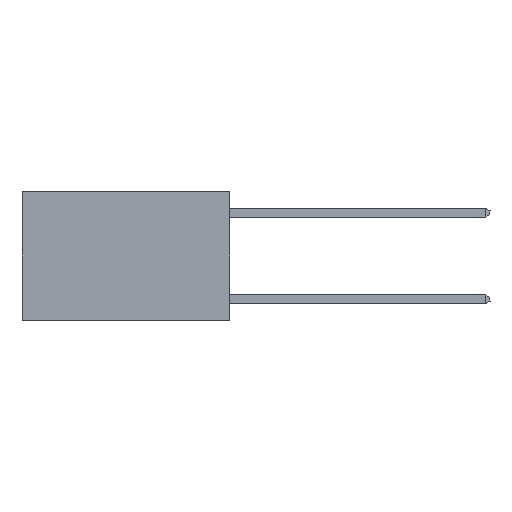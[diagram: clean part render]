
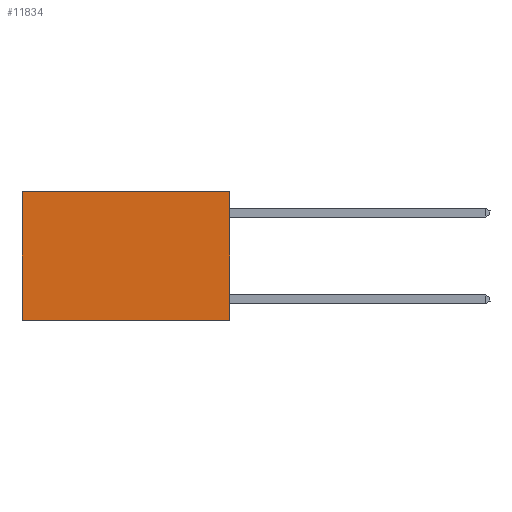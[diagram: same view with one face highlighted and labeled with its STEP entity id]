
A CAD part, left-side view. The second image highlights one B-rep face of the part: STEP entity #11834.
In plain terms, the highlighted planar face has unit normal (-1, 0, 0).
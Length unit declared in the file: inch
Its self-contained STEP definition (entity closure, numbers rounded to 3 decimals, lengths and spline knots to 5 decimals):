
#857 = LINE ( 'NONE', #11446, #1063 ) ;
#1063 = VECTOR ( 'NONE', #11512, 39.37008 ) ;
#1715 = VERTEX_POINT ( 'NONE', #8398 ) ;
#2394 = CARTESIAN_POINT ( 'NONE',  ( 0.2625, 0.6, 0. ) ) ;
#2595 = DIRECTION ( 'NONE',  ( 0., 0., -1. ) ) ;
#2798 = DIRECTION ( 'NONE',  ( 0., 1., 0. ) ) ;
#3141 = VERTEX_POINT ( 'NONE', #9668 ) ;
#3195 = VERTEX_POINT ( 'NONE', #3634 ) ;
#3634 = CARTESIAN_POINT ( 'NONE',  ( 0.2625, 0., 0. ) ) ;
#4478 = ORIENTED_EDGE ( 'NONE', *, *, #11372, .T. ) ;
#4837 = ORIENTED_EDGE ( 'NONE', *, *, #5421, .F. ) ;
#5124 = ORIENTED_EDGE ( 'NONE', *, *, #5441, .F. ) ;
#5239 = LINE ( 'NONE', #9441, #12549 ) ;
#5377 = VECTOR ( 'NONE', #2595, 39.37008 ) ;
#5421 = EDGE_CURVE ( 'NONE', #1715, #9700, #5239, .T. ) ;
#5441 = EDGE_CURVE ( 'NONE', #3195, #1715, #9586, .T. ) ;
#5801 = LINE ( 'NONE', #2394, #5377 ) ;
#6677 = PLANE ( 'NONE',  #11346 ) ;
#7125 = EDGE_CURVE ( 'NONE', #3195, #3141, #857, .T. ) ;
#8398 = CARTESIAN_POINT ( 'NONE',  ( 0.2625, 0., -0.37 ) ) ;
#8776 = EDGE_LOOP ( 'NONE', ( #4478, #4837, #5124, #10628 ) ) ;
#9065 = CARTESIAN_POINT ( 'NONE',  ( 0.2625, 0.6, -0.37 ) ) ;
#9441 = CARTESIAN_POINT ( 'NONE',  ( 0.2625, 0., -0.37 ) ) ;
#9586 = LINE ( 'NONE', #10565, #10103 ) ;
#9668 = CARTESIAN_POINT ( 'NONE',  ( 0.2625, 0.6, 0. ) ) ;
#9700 = VERTEX_POINT ( 'NONE', #9065 ) ;
#10103 = VECTOR ( 'NONE', #12846, 39.37008 ) ;
#10565 = CARTESIAN_POINT ( 'NONE',  ( 0.2625, 0., 0. ) ) ;
#10628 = ORIENTED_EDGE ( 'NONE', *, *, #7125, .T. ) ;
#10790 = DIRECTION ( 'NONE',  ( 1., 0., 0. ) ) ;
#10917 = DIRECTION ( 'NONE',  ( 0., 0., -1. ) ) ;
#11346 = AXIS2_PLACEMENT_3D ( 'NONE', #12937, #10790, #10917 ) ;
#11372 = EDGE_CURVE ( 'NONE', #3141, #9700, #5801, .T. ) ;
#11446 = CARTESIAN_POINT ( 'NONE',  ( 0.2625, 0., 0. ) ) ;
#11512 = DIRECTION ( 'NONE',  ( 0., 1., 0. ) ) ;
#11834 = ADVANCED_FACE ( 'NONE', ( #13000 ), #6677, .F. ) ;
#12549 = VECTOR ( 'NONE', #2798, 39.37008 ) ;
#12846 = DIRECTION ( 'NONE',  ( 0., 0., -1. ) ) ;
#12937 = CARTESIAN_POINT ( 'NONE',  ( 0.2625, 0., 0. ) ) ;
#13000 = FACE_OUTER_BOUND ( 'NONE', #8776, .T. ) ;
